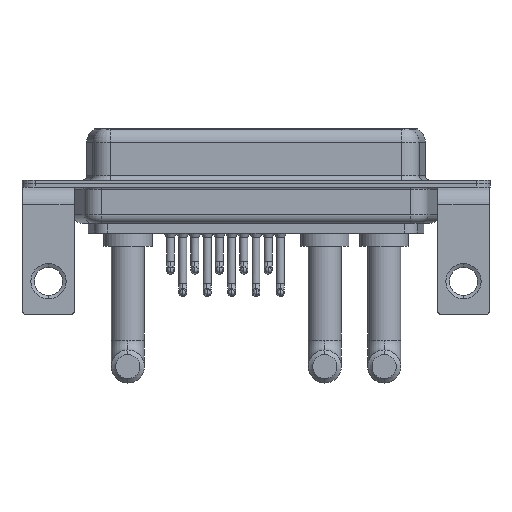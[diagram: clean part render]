
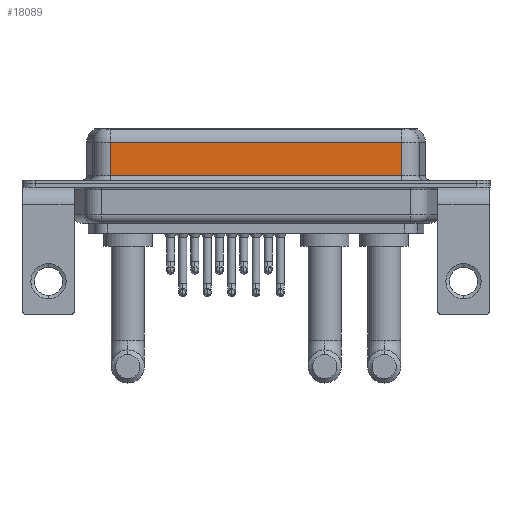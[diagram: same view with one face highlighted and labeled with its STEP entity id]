
A CAD part, front view. The second image highlights one B-rep face of the part: STEP entity #18089.
In plain terms, the highlighted planar face has unit normal (0, -1, 0).
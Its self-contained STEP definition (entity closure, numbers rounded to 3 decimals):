
#94 = DIRECTION ( 'NONE',  ( 0., 0., -1. ) ) ;
#108 = LINE ( 'NONE', #6188, #4458 ) ;
#317 = CARTESIAN_POINT ( 'NONE',  ( 40.037, -3.95, 4.65 ) ) ;
#2330 = CARTESIAN_POINT ( 'NONE',  ( 7.013, -3.95, 0.9 ) ) ;
#2714 = CARTESIAN_POINT ( 'NONE',  ( 7.013, -3.95, 4.65 ) ) ;
#3828 = DIRECTION ( 'NONE',  ( 1., 0., 0. ) ) ;
#4035 = VERTEX_POINT ( 'NONE', #19377 ) ;
#4458 = VECTOR ( 'NONE', #12288, 1000. ) ;
#4690 = DIRECTION ( 'NONE',  ( 0., 1., 0. ) ) ;
#4723 = EDGE_CURVE ( 'NONE', #4035, #10126, #108, .T. ) ;
#5498 = ORIENTED_EDGE ( 'NONE', *, *, #16811, .T. ) ;
#6188 = CARTESIAN_POINT ( 'NONE',  ( 40.037, -3.95, 6.4 ) ) ;
#6284 = FACE_OUTER_BOUND ( 'NONE', #13413, .T. ) ;
#7198 = EDGE_CURVE ( 'NONE', #4035, #10696, #10783, .T. ) ;
#7859 = CARTESIAN_POINT ( 'NONE',  ( 7.013, -3.95, 6.4 ) ) ;
#8810 = ORIENTED_EDGE ( 'NONE', *, *, #4723, .F. ) ;
#8940 = VECTOR ( 'NONE', #10590, 1000. ) ;
#10126 = VERTEX_POINT ( 'NONE', #11046 ) ;
#10179 = VECTOR ( 'NONE', #3828, 1000. ) ;
#10230 = VERTEX_POINT ( 'NONE', #2330 ) ;
#10590 = DIRECTION ( 'NONE',  ( -1., 0., 0. ) ) ;
#10696 = VERTEX_POINT ( 'NONE', #2714 ) ;
#10783 = LINE ( 'NONE', #317, #8940 ) ;
#10877 = DIRECTION ( 'NONE',  ( 0., 0., 1. ) ) ;
#11046 = CARTESIAN_POINT ( 'NONE',  ( 40.037, -3.95, 0.9 ) ) ;
#11180 = ORIENTED_EDGE ( 'NONE', *, *, #7198, .T. ) ;
#11354 = ORIENTED_EDGE ( 'NONE', *, *, #12633, .T. ) ;
#12288 = DIRECTION ( 'NONE',  ( 0., 0., -1. ) ) ;
#12633 = EDGE_CURVE ( 'NONE', #10696, #10230, #13787, .T. ) ;
#13030 = CARTESIAN_POINT ( 'NONE',  ( 40.037, -3.95, 0.9 ) ) ;
#13413 = EDGE_LOOP ( 'NONE', ( #8810, #11180, #11354, #5498 ) ) ;
#13787 = LINE ( 'NONE', #7859, #14225 ) ;
#14225 = VECTOR ( 'NONE', #94, 1000. ) ;
#14342 = LINE ( 'NONE', #13030, #10179 ) ;
#15796 = PLANE ( 'NONE',  #16639 ) ;
#16639 = AXIS2_PLACEMENT_3D ( 'NONE', #18739, #4690, #10877 ) ;
#16811 = EDGE_CURVE ( 'NONE', #10230, #10126, #14342, .T. ) ;
#18089 = ADVANCED_FACE ( 'NONE', ( #6284 ), #15796, .F. ) ;
#18739 = CARTESIAN_POINT ( 'NONE',  ( 40.037, -3.95, 6.4 ) ) ;
#19377 = CARTESIAN_POINT ( 'NONE',  ( 40.037, -3.95, 4.65 ) ) ;
